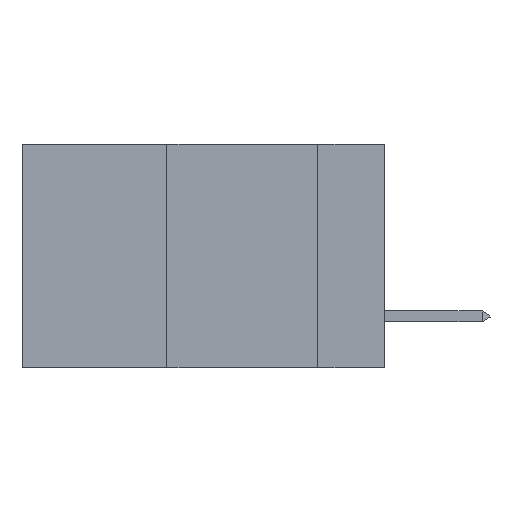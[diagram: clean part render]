
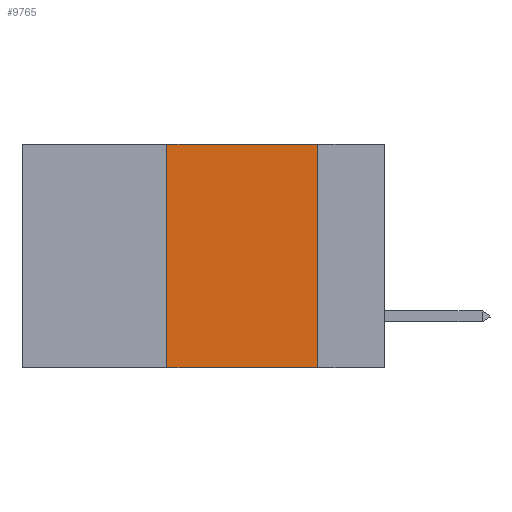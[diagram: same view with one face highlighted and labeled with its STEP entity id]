
A CAD part, left-side view. The second image highlights one B-rep face of the part: STEP entity #9765.
In plain terms, the highlighted planar face has unit normal (-1, 0, 0).
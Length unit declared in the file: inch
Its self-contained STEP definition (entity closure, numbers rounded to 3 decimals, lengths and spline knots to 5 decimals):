
#626 = CARTESIAN_POINT ( 'NONE',  ( 0., 0.11, 0. ) ) ;
#1684 = EDGE_CURVE ( 'NONE', #10521, #2826, #16454, .T. ) ;
#2730 = ORIENTED_EDGE ( 'NONE', *, *, #16684, .T. ) ;
#2826 = VERTEX_POINT ( 'NONE', #4036 ) ;
#3887 = VECTOR ( 'NONE', #11401, 39.37008 ) ;
#4036 = CARTESIAN_POINT ( 'NONE',  ( 0., 0.11, -0.37 ) ) ;
#4326 = LINE ( 'NONE', #25290, #3887 ) ;
#4377 = CARTESIAN_POINT ( 'NONE',  ( 0., 0.36, -0.37 ) ) ;
#4489 = CARTESIAN_POINT ( 'NONE',  ( 0., 0.6, 0. ) ) ;
#4637 = VECTOR ( 'NONE', #17249, 39.37008 ) ;
#6547 = FACE_OUTER_BOUND ( 'NONE', #25182, .T. ) ;
#6675 = LINE ( 'NONE', #13406, #12596 ) ;
#7765 = LINE ( 'NONE', #4489, #12720 ) ;
#7796 = EDGE_CURVE ( 'NONE', #9197, #12998, #6675, .T. ) ;
#9197 = VERTEX_POINT ( 'NONE', #4377 ) ;
#9765 = ADVANCED_FACE ( 'NONE', ( #6547 ), #17237, .F. ) ;
#10129 = AXIS2_PLACEMENT_3D ( 'NONE', #11706, #23841, #21009 ) ;
#10521 = VERTEX_POINT ( 'NONE', #626 ) ;
#11401 = DIRECTION ( 'NONE',  ( 0., -1., 0. ) ) ;
#11706 = CARTESIAN_POINT ( 'NONE',  ( 0., 0.6, 0. ) ) ;
#12596 = VECTOR ( 'NONE', #17378, 39.37008 ) ;
#12720 = VECTOR ( 'NONE', #18506, 39.37008 ) ;
#12998 = VERTEX_POINT ( 'NONE', #20405 ) ;
#13406 = CARTESIAN_POINT ( 'NONE',  ( 0., 0.36, 0. ) ) ;
#14043 = EDGE_CURVE ( 'NONE', #12998, #10521, #7765, .T. ) ;
#15028 = ORIENTED_EDGE ( 'NONE', *, *, #7796, .F. ) ;
#15377 = ORIENTED_EDGE ( 'NONE', *, *, #1684, .F. ) ;
#16454 = LINE ( 'NONE', #23077, #4637 ) ;
#16684 = EDGE_CURVE ( 'NONE', #9197, #2826, #4326, .T. ) ;
#17237 = PLANE ( 'NONE',  #10129 ) ;
#17249 = DIRECTION ( 'NONE',  ( 0., 0., -1. ) ) ;
#17378 = DIRECTION ( 'NONE',  ( 0., 0., 1. ) ) ;
#18506 = DIRECTION ( 'NONE',  ( 0., -1., 0. ) ) ;
#20405 = CARTESIAN_POINT ( 'NONE',  ( 0., 0.36, 0. ) ) ;
#21009 = DIRECTION ( 'NONE',  ( 0., 0., -1. ) ) ;
#22526 = ORIENTED_EDGE ( 'NONE', *, *, #14043, .F. ) ;
#23077 = CARTESIAN_POINT ( 'NONE',  ( 0., 0.11, 0. ) ) ;
#23841 = DIRECTION ( 'NONE',  ( 1., 0., 0. ) ) ;
#25182 = EDGE_LOOP ( 'NONE', ( #15377, #22526, #15028, #2730 ) ) ;
#25290 = CARTESIAN_POINT ( 'NONE',  ( 0., 0.6, -0.37 ) ) ;
